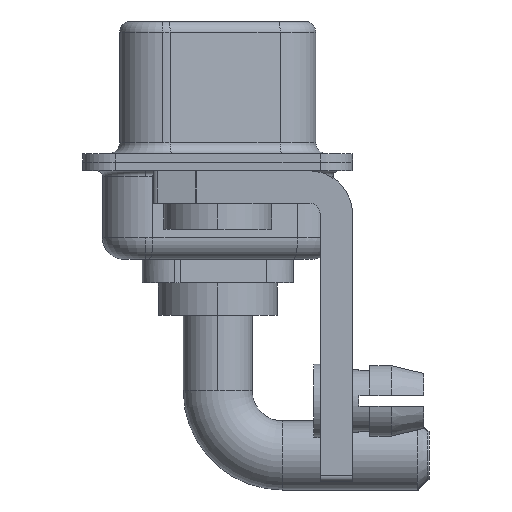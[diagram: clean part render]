
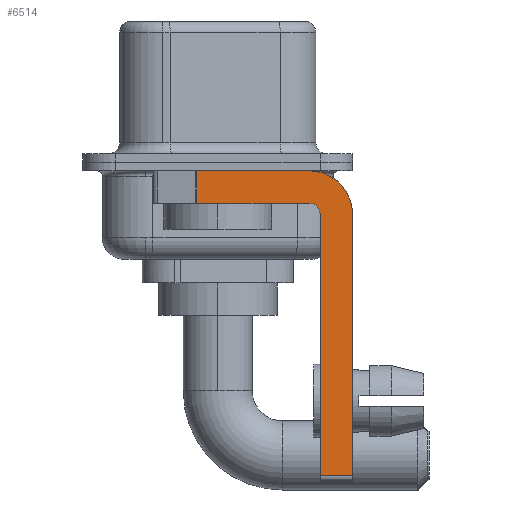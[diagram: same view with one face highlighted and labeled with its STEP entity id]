
A CAD part, left-side view. The second image highlights one B-rep face of the part: STEP entity #6514.
In plain terms, the highlighted planar face has unit normal (-1, 0, 0).
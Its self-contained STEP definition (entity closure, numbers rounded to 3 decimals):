
#253 = ORIENTED_EDGE ( 'NONE', *, *, #11494, .F. ) ;
#1305 = ORIENTED_EDGE ( 'NONE', *, *, #8297, .T. ) ;
#1362 = DIRECTION ( 'NONE',  ( 0., 0., -1. ) ) ;
#1433 = CARTESIAN_POINT ( 'NONE',  ( -2.9, -4.75, -14.55 ) ) ;
#2324 = EDGE_LOOP ( 'NONE', ( #14801, #1305, #15106, #8833, #253, #11143, #8120, #7183 ) ) ;
#2327 = DIRECTION ( 'NONE',  ( -1., 0., 0. ) ) ;
#2415 = CARTESIAN_POINT ( 'NONE',  ( -2.9, 3., -0.4 ) ) ;
#2450 = CARTESIAN_POINT ( 'NONE',  ( -2.9, -4.25, -14.55 ) ) ;
#2585 = VERTEX_POINT ( 'NONE', #16628 ) ;
#2704 = CARTESIAN_POINT ( 'NONE',  ( -2.9, -4.25, -2.4 ) ) ;
#3085 = CARTESIAN_POINT ( 'NONE',  ( -2.9, -6.25, -2.4 ) ) ;
#3418 = VECTOR ( 'NONE', #16662, 1000. ) ;
#3979 = EDGE_CURVE ( 'NONE', #4853, #10791, #10587, .T. ) ;
#4370 = LINE ( 'NONE', #12339, #11177 ) ;
#4853 = VERTEX_POINT ( 'NONE', #12426 ) ;
#5013 = LINE ( 'NONE', #9918, #3418 ) ;
#5074 = VERTEX_POINT ( 'NONE', #12164 ) ;
#5279 = DIRECTION ( 'NONE',  ( 0., 0., -1. ) ) ;
#5450 = DIRECTION ( 'NONE',  ( 1., 0., 0. ) ) ;
#5726 = VERTEX_POINT ( 'NONE', #3085 ) ;
#5822 = VERTEX_POINT ( 'NONE', #12764 ) ;
#5949 = CARTESIAN_POINT ( 'NONE',  ( -2.9, -4.75, -2.4 ) ) ;
#6085 = AXIS2_PLACEMENT_3D ( 'NONE', #2704, #5450, #6727 ) ;
#6514 = ADVANCED_FACE ( 'NONE', ( #10428 ), #9410, .F. ) ;
#6727 = DIRECTION ( 'NONE',  ( 0., 0., -1. ) ) ;
#7183 = ORIENTED_EDGE ( 'NONE', *, *, #11853, .F. ) ;
#7408 = EDGE_CURVE ( 'NONE', #15060, #4853, #15746, .T. ) ;
#7554 = DIRECTION ( 'NONE',  ( 0., 0., 1. ) ) ;
#7616 = EDGE_CURVE ( 'NONE', #5074, #2585, #8041, .T. ) ;
#7968 = CARTESIAN_POINT ( 'NONE',  ( -2.9, -4.25, -2.4 ) ) ;
#8041 = LINE ( 'NONE', #2415, #11066 ) ;
#8120 = ORIENTED_EDGE ( 'NONE', *, *, #14195, .F. ) ;
#8126 = DIRECTION ( 'NONE',  ( 0., -1., 0. ) ) ;
#8297 = EDGE_CURVE ( 'NONE', #5074, #10791, #5013, .T. ) ;
#8833 = ORIENTED_EDGE ( 'NONE', *, *, #7408, .F. ) ;
#9410 = PLANE ( 'NONE',  #6085 ) ;
#9918 = CARTESIAN_POINT ( 'NONE',  ( -2.9, 0.978, -1.9 ) ) ;
#10274 = VECTOR ( 'NONE', #5279, 1000. ) ;
#10327 = CARTESIAN_POINT ( 'NONE',  ( -2.9, 0.978, -1.9 ) ) ;
#10428 = FACE_OUTER_BOUND ( 'NONE', #2324, .T. ) ;
#10572 = VECTOR ( 'NONE', #14174, 1000. ) ;
#10587 = LINE ( 'NONE', #16824, #13607 ) ;
#10733 = DIRECTION ( 'NONE',  ( 0., 0., 1. ) ) ;
#10791 = VERTEX_POINT ( 'NONE', #10327 ) ;
#11066 = VECTOR ( 'NONE', #8126, 1000. ) ;
#11143 = ORIENTED_EDGE ( 'NONE', *, *, #14602, .T. ) ;
#11177 = VECTOR ( 'NONE', #10733, 1000. ) ;
#11458 = CIRCLE ( 'NONE', #13106, 2. ) ;
#11494 = EDGE_CURVE ( 'NONE', #13974, #15060, #4370, .T. ) ;
#11580 = DIRECTION ( 'NONE',  ( 1., 0., 0. ) ) ;
#11620 = CARTESIAN_POINT ( 'NONE',  ( -2.9, -6.25, -2.4 ) ) ;
#11853 = EDGE_CURVE ( 'NONE', #2585, #5726, #11458, .T. ) ;
#12164 = CARTESIAN_POINT ( 'NONE',  ( -2.9, 0.978, -0.4 ) ) ;
#12339 = CARTESIAN_POINT ( 'NONE',  ( -2.9, -4.75, -14.8 ) ) ;
#12426 = CARTESIAN_POINT ( 'NONE',  ( -2.9, -4.25, -1.9 ) ) ;
#12764 = CARTESIAN_POINT ( 'NONE',  ( -2.9, -6.25, -14.55 ) ) ;
#13065 = DIRECTION ( 'NONE',  ( 0., 1., 0. ) ) ;
#13106 = AXIS2_PLACEMENT_3D ( 'NONE', #7968, #11580, #1362 ) ;
#13288 = AXIS2_PLACEMENT_3D ( 'NONE', #16635, #2327, #7554 ) ;
#13607 = VECTOR ( 'NONE', #13065, 1000. ) ;
#13841 = LINE ( 'NONE', #2450, #10572 ) ;
#13974 = VERTEX_POINT ( 'NONE', #1433 ) ;
#14174 = DIRECTION ( 'NONE',  ( 0., -1., 0. ) ) ;
#14195 = EDGE_CURVE ( 'NONE', #5726, #5822, #16914, .T. ) ;
#14602 = EDGE_CURVE ( 'NONE', #13974, #5822, #13841, .T. ) ;
#14801 = ORIENTED_EDGE ( 'NONE', *, *, #7616, .F. ) ;
#15060 = VERTEX_POINT ( 'NONE', #5949 ) ;
#15106 = ORIENTED_EDGE ( 'NONE', *, *, #3979, .F. ) ;
#15746 = CIRCLE ( 'NONE', #13288, 0.5 ) ;
#16628 = CARTESIAN_POINT ( 'NONE',  ( -2.9, -4.25, -0.4 ) ) ;
#16635 = CARTESIAN_POINT ( 'NONE',  ( -2.9, -4.25, -2.4 ) ) ;
#16662 = DIRECTION ( 'NONE',  ( 0., 0., -1. ) ) ;
#16824 = CARTESIAN_POINT ( 'NONE',  ( -2.9, -4.25, -1.9 ) ) ;
#16914 = LINE ( 'NONE', #11620, #10274 ) ;
